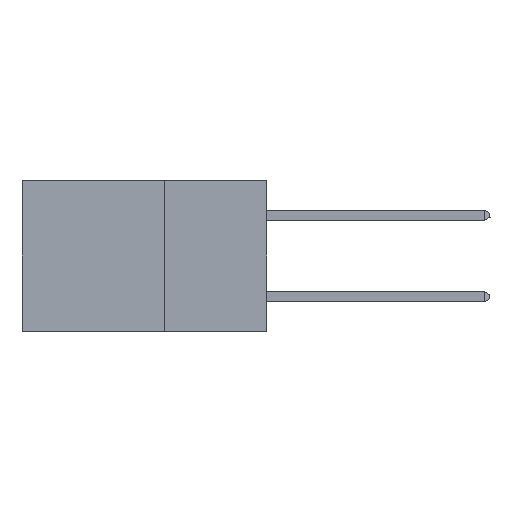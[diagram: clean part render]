
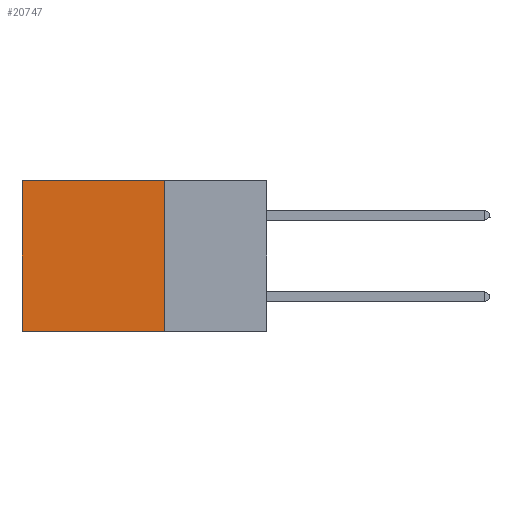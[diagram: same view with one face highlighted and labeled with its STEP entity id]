
A CAD part, left-side view. The second image highlights one B-rep face of the part: STEP entity #20747.
In plain terms, the highlighted planar face has unit normal (-1, 0, 0).
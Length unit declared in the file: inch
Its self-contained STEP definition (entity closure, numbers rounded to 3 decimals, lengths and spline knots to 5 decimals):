
#1190 = EDGE_CURVE ( 'NONE', #22445, #35814, #24794, .T. ) ;
#1805 = PLANE ( 'NONE',  #4098 ) ;
#2254 = ORIENTED_EDGE ( 'NONE', *, *, #7867, .T. ) ;
#3015 = ORIENTED_EDGE ( 'NONE', *, *, #22113, .F. ) ;
#4098 = AXIS2_PLACEMENT_3D ( 'NONE', #19783, #36458, #5627 ) ;
#5627 = DIRECTION ( 'NONE',  ( 0., 0., -1. ) ) ;
#6339 = VECTOR ( 'NONE', #23318, 39.37008 ) ;
#7701 = DIRECTION ( 'NONE',  ( 0., 1., 0. ) ) ;
#7867 = EDGE_CURVE ( 'NONE', #35814, #36020, #11253, .T. ) ;
#10030 = LINE ( 'NONE', #26692, #6339 ) ;
#11253 = LINE ( 'NONE', #27677, #39657 ) ;
#11600 = CARTESIAN_POINT ( 'NONE',  ( 0.2875, 0.6, -0.37 ) ) ;
#12201 = LINE ( 'NONE', #25937, #23484 ) ;
#12963 = VECTOR ( 'NONE', #7701, 39.37008 ) ;
#13283 = EDGE_LOOP ( 'NONE', ( #2254, #3015, #17197, #41434 ) ) ;
#17197 = ORIENTED_EDGE ( 'NONE', *, *, #32794, .F. ) ;
#19413 = CARTESIAN_POINT ( 'NONE',  ( 0.2875, 0.25, -0.37 ) ) ;
#19783 = CARTESIAN_POINT ( 'NONE',  ( 0.2875, 0.25, 0. ) ) ;
#20196 = VERTEX_POINT ( 'NONE', #19413 ) ;
#20747 = ADVANCED_FACE ( 'NONE', ( #29237 ), #1805, .F. ) ;
#22113 = EDGE_CURVE ( 'NONE', #20196, #36020, #12201, .T. ) ;
#22445 = VERTEX_POINT ( 'NONE', #40015 ) ;
#23318 = DIRECTION ( 'NONE',  ( 0., 0., -1. ) ) ;
#23484 = VECTOR ( 'NONE', #39681, 39.37008 ) ;
#24794 = LINE ( 'NONE', #38529, #12963 ) ;
#25937 = CARTESIAN_POINT ( 'NONE',  ( 0.2875, 0.25, -0.37 ) ) ;
#26692 = CARTESIAN_POINT ( 'NONE',  ( 0.2875, 0.25, 0. ) ) ;
#27677 = CARTESIAN_POINT ( 'NONE',  ( 0.2875, 0.6, 0. ) ) ;
#28132 = DIRECTION ( 'NONE',  ( 0., 0., -1. ) ) ;
#29237 = FACE_OUTER_BOUND ( 'NONE', #13283, .T. ) ;
#32794 = EDGE_CURVE ( 'NONE', #22445, #20196, #10030, .T. ) ;
#35814 = VERTEX_POINT ( 'NONE', #37962 ) ;
#36020 = VERTEX_POINT ( 'NONE', #11600 ) ;
#36458 = DIRECTION ( 'NONE',  ( 1., 0., 0. ) ) ;
#37962 = CARTESIAN_POINT ( 'NONE',  ( 0.2875, 0.6, 0. ) ) ;
#38529 = CARTESIAN_POINT ( 'NONE',  ( 0.2875, 0.25, 0. ) ) ;
#39657 = VECTOR ( 'NONE', #28132, 39.37008 ) ;
#39681 = DIRECTION ( 'NONE',  ( 0., 1., 0. ) ) ;
#40015 = CARTESIAN_POINT ( 'NONE',  ( 0.2875, 0.25, 0. ) ) ;
#41434 = ORIENTED_EDGE ( 'NONE', *, *, #1190, .T. ) ;
